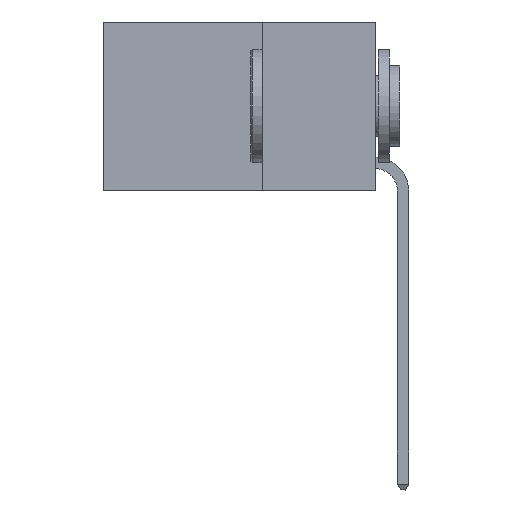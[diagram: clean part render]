
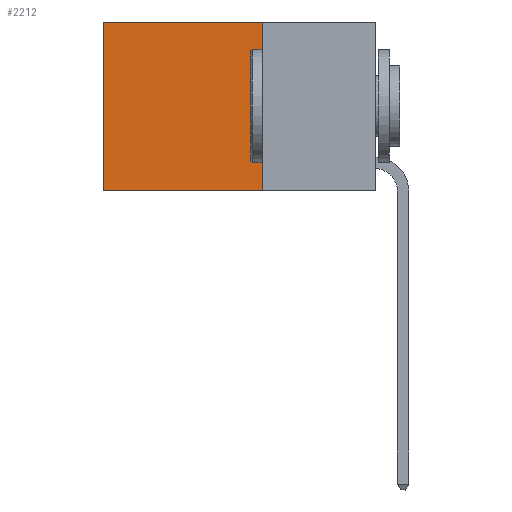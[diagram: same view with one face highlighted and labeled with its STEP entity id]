
A CAD part, left-side view. The second image highlights one B-rep face of the part: STEP entity #2212.
In plain terms, the highlighted planar face has unit normal (-1, 0, 0).
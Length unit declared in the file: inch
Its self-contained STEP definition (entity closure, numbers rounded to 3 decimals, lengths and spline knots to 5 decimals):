
#107 = ORIENTED_EDGE ( 'NONE', *, *, #12568, .F. ) ;
#949 = ORIENTED_EDGE ( 'NONE', *, *, #15423, .T. ) ;
#1071 = CARTESIAN_POINT ( 'NONE',  ( 0.2625, 0.25, 0. ) ) ;
#1722 = EDGE_CURVE ( 'NONE', #12770, #13484, #5396, .T. ) ;
#1752 = CARTESIAN_POINT ( 'NONE',  ( 0.2625, 0.6, 0. ) ) ;
#1795 = VECTOR ( 'NONE', #7106, 39.37008 ) ;
#1840 = LINE ( 'NONE', #9956, #15115 ) ;
#2212 = ADVANCED_FACE ( 'NONE', ( #8103 ), #10436, .F. ) ;
#3176 = ORIENTED_EDGE ( 'NONE', *, *, #1722, .F. ) ;
#4499 = DIRECTION ( 'NONE',  ( 0., 1., 0. ) ) ;
#4739 = LINE ( 'NONE', #9123, #8311 ) ;
#5119 = DIRECTION ( 'NONE',  ( 0., 0., -1. ) ) ;
#5396 = LINE ( 'NONE', #7313, #1795 ) ;
#5846 = VERTEX_POINT ( 'NONE', #1752 ) ;
#6694 = AXIS2_PLACEMENT_3D ( 'NONE', #7700, #13080, #5119 ) ;
#6722 = VECTOR ( 'NONE', #4499, 39.37008 ) ;
#7106 = DIRECTION ( 'NONE',  ( 0., 0., -1. ) ) ;
#7129 = LINE ( 'NONE', #11159, #6722 ) ;
#7313 = CARTESIAN_POINT ( 'NONE',  ( 0.2625, 0.25, 0. ) ) ;
#7700 = CARTESIAN_POINT ( 'NONE',  ( 0.2625, 0.25, 0. ) ) ;
#8065 = EDGE_CURVE ( 'NONE', #5846, #9447, #4739, .T. ) ;
#8103 = FACE_OUTER_BOUND ( 'NONE', #14659, .T. ) ;
#8311 = VECTOR ( 'NONE', #10933, 39.37008 ) ;
#8719 = CARTESIAN_POINT ( 'NONE',  ( 0.2625, 0.6, -0.37 ) ) ;
#9123 = CARTESIAN_POINT ( 'NONE',  ( 0.2625, 0.6, 0. ) ) ;
#9447 = VERTEX_POINT ( 'NONE', #8719 ) ;
#9956 = CARTESIAN_POINT ( 'NONE',  ( 0.2625, 0.25, -0.37 ) ) ;
#10436 = PLANE ( 'NONE',  #6694 ) ;
#10438 = ORIENTED_EDGE ( 'NONE', *, *, #8065, .T. ) ;
#10933 = DIRECTION ( 'NONE',  ( 0., 0., -1. ) ) ;
#11159 = CARTESIAN_POINT ( 'NONE',  ( 0.2625, 0.25, 0. ) ) ;
#11288 = DIRECTION ( 'NONE',  ( 0., 1., 0. ) ) ;
#12568 = EDGE_CURVE ( 'NONE', #13484, #9447, #1840, .T. ) ;
#12770 = VERTEX_POINT ( 'NONE', #1071 ) ;
#13080 = DIRECTION ( 'NONE',  ( 1., 0., 0. ) ) ;
#13484 = VERTEX_POINT ( 'NONE', #13487 ) ;
#13487 = CARTESIAN_POINT ( 'NONE',  ( 0.2625, 0.25, -0.37 ) ) ;
#14659 = EDGE_LOOP ( 'NONE', ( #10438, #107, #3176, #949 ) ) ;
#15115 = VECTOR ( 'NONE', #11288, 39.37008 ) ;
#15423 = EDGE_CURVE ( 'NONE', #12770, #5846, #7129, .T. ) ;
